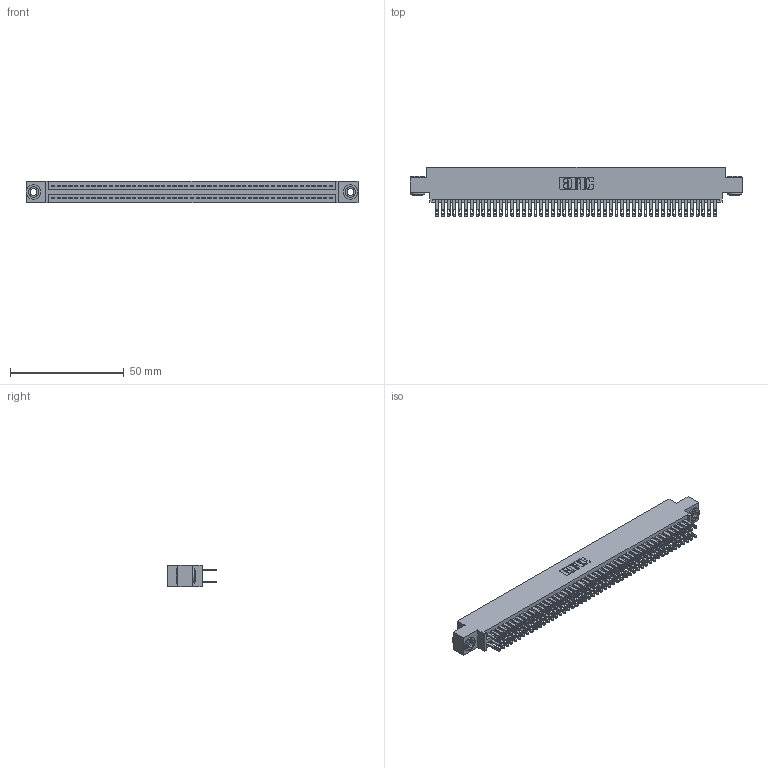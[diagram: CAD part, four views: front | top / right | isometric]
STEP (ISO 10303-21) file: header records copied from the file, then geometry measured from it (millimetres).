
FILE_DESCRIPTION (( 'STEP AP203' ), '1' );
FILE_NAME ('345-098-500-803.STEP', '2018-10-05T07:48:51', ( '' ), ( '' ), 'SwSTEP 2.0', 'SolidWorks 2016', '' );
FILE_SCHEMA (( 'CONFIG_CONTROL_DESIGN' ));
Length unit declared in the file: inch
Products named in the file (4): 345 Part_0.170 Offset - 0.156 Dia-TH; 345-250-002_345-250-002-102; 345-292-001_345-293-100; 345-098-500-803
Assembly tree (101 placements, depth 2):
  345-098-500-803
    345 Part_0.170 Offset - 0.156 Dia-TH
    345-292-001_345-293-100  x98
    345-250-002_345-250-002-102  x2
Bounding box: 145.67 x 21.51 x 9.4 mm (x, y, z)
Volume: 14420.9 mm3; surface area: 22800 mm2
Topology: 101 solids, 101 shells, 4676 faces, 14247 edges, 9494 vertices
Faces by surface type: plane 2740, cylinder 1928, cone 8
Entity records: 38216 total; most frequent: CARTESIAN_POINT 6375, ORIENTED_EDGE 6302, DIRECTION 5645, EDGE_CURVE 3151, VECTOR 2795, LINE 2795, VERTEX_POINT 2098, AXIS2_PLACEMENT_3D 1425
